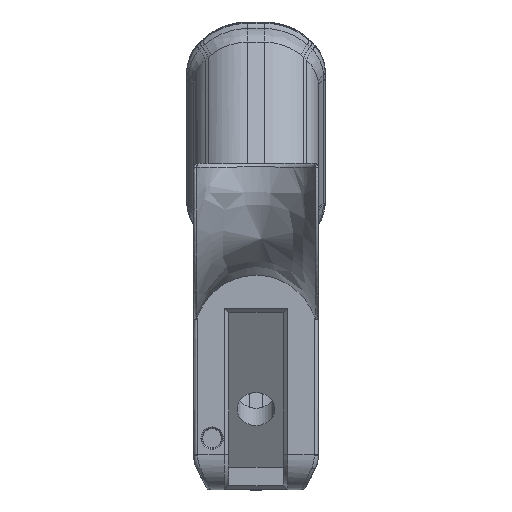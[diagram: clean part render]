
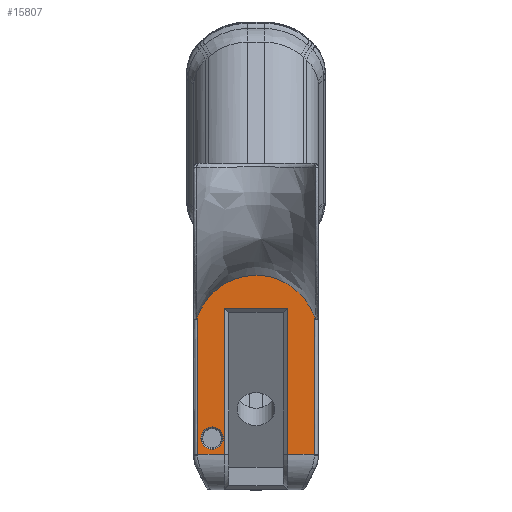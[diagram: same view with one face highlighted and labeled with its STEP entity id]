
A CAD part, top view. The second image highlights one B-rep face of the part: STEP entity #15807.
In plain terms, the highlighted planar face has unit normal (0, 0, 1).
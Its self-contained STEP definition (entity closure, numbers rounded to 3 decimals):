
#673=B_SPLINE_CURVE_WITH_KNOTS('',3,(#37954,#37955,#37956,#37957,#37958,
#37959,#37960,#37961,#37962,#37963,#37964,#37965),.UNSPECIFIED.,.F.,.F.,
(4,2,2,2,2,4),(1.71,1.762,2.19,2.624,
3.022,3.106),.UNSPECIFIED.);
#674=B_SPLINE_CURVE_WITH_KNOTS('',3,(#37967,#37968,#37969,#37970,#37971,
#37972,#37973,#37974,#37975,#37976),.UNSPECIFIED.,.F.,.F.,(4,2,2,2,4),(0.313,
0.444,0.89,1.331,1.71),
 .UNSPECIFIED.);
#727=B_SPLINE_CURVE_WITH_KNOTS('',3,(#39650,#39651,#39652,#39653),
 .UNSPECIFIED.,.F.,.F.,(4,4),(-2.445,-0.005),
 .UNSPECIFIED.);
#729=B_SPLINE_CURVE_WITH_KNOTS('',3,(#39761,#39762,#39763,#39764),
 .UNSPECIFIED.,.F.,.F.,(4,4),(-7.406,-4.966),
 .UNSPECIFIED.);
#1639=FACE_BOUND('',#4707,.T.);
#2454=CIRCLE('',#17283,2.);
#3603=FACE_OUTER_BOUND('',#4706,.T.);
#4706=EDGE_LOOP('',(#14201,#14202,#14203,#14204,#14205,#14206,#14207,#14208,
#14209));
#4707=EDGE_LOOP('',(#14210));
#5472=LINE('',#37829,#6207);
#5478=LINE('',#37840,#6213);
#5483=LINE('',#37858,#6218);
#5490=LINE('',#39758,#6225);
#5491=LINE('',#39760,#6226);
#6207=VECTOR('',#20745,10.);
#6213=VECTOR('',#20755,10.);
#6218=VECTOR('',#20768,10.);
#6225=VECTOR('',#20829,10.);
#6226=VECTOR('',#20830,10.);
#7397=VERTEX_POINT('',#37827);
#7398=VERTEX_POINT('',#37828);
#7401=VERTEX_POINT('',#37839);
#7405=VERTEX_POINT('',#37857);
#7412=VERTEX_POINT('',#37948);
#7413=VERTEX_POINT('',#37953);
#7414=VERTEX_POINT('',#37966);
#7460=VERTEX_POINT('',#39757);
#7461=VERTEX_POINT('',#39759);
#7462=VERTEX_POINT('',#39765);
#9639=EDGE_CURVE('',#7397,#7398,#5472,.T.);
#9645=EDGE_CURVE('',#7401,#7397,#5478,.T.);
#9652=EDGE_CURVE('',#7405,#7398,#5483,.T.);
#9660=EDGE_CURVE('',#7413,#7412,#673,.T.);
#9661=EDGE_CURVE('',#7414,#7413,#674,.T.);
#9738=EDGE_CURVE('',#7405,#7412,#727,.T.);
#9740=EDGE_CURVE('',#7460,#7401,#5490,.T.);
#9741=EDGE_CURVE('',#7461,#7460,#5491,.T.);
#9742=EDGE_CURVE('',#7414,#7461,#729,.T.);
#9743=EDGE_CURVE('',#7462,#7462,#2454,.T.);
#14201=ORIENTED_EDGE('',*,*,#9660,.T.);
#14202=ORIENTED_EDGE('',*,*,#9738,.F.);
#14203=ORIENTED_EDGE('',*,*,#9652,.T.);
#14204=ORIENTED_EDGE('',*,*,#9639,.F.);
#14205=ORIENTED_EDGE('',*,*,#9645,.F.);
#14206=ORIENTED_EDGE('',*,*,#9740,.F.);
#14207=ORIENTED_EDGE('',*,*,#9741,.F.);
#14208=ORIENTED_EDGE('',*,*,#9742,.F.);
#14209=ORIENTED_EDGE('',*,*,#9661,.T.);
#14210=ORIENTED_EDGE('',*,*,#9743,.F.);
#14774=PLANE('',#17282);
#15807=ADVANCED_FACE('',(#3603,#1639),#14774,.T.);
#17282=AXIS2_PLACEMENT_3D('',#39756,#20827,#20828);
#17283=AXIS2_PLACEMENT_3D('',#39766,#20831,#20832);
#20745=DIRECTION('',(0.,-1.,0.));
#20755=DIRECTION('',(-1.,0.,0.));
#20768=DIRECTION('',(1.,0.,0.));
#20827=DIRECTION('center_axis',(0.,0.,
1.));
#20828=DIRECTION('ref_axis',(0.,-1.,0.));
#20829=DIRECTION('',(0.,1.,0.));
#20830=DIRECTION('',(-1.,0.,0.));
#20831=DIRECTION('center_axis',(0.,0.,
1.));
#20832=DIRECTION('ref_axis',(1.,0.,0.));
#37827=CARTESIAN_POINT('',(18.417,-117.318,28.406));
#37828=CARTESIAN_POINT('',(18.417,-143.468,28.406));
#37829=CARTESIAN_POINT('',(18.417,-114.618,28.406));
#37839=CARTESIAN_POINT('',(29.746,-117.318,28.406));
#37840=CARTESIAN_POINT('',(24.173,-117.318,28.406));
#37857=CARTESIAN_POINT('',(13.65,-143.468,28.406));
#37858=CARTESIAN_POINT('',(28.956,-143.468,28.406));
#37948=CARTESIAN_POINT('',(13.518,-119.073,28.406));
#37953=CARTESIAN_POINT('',(24.081,-111.416,28.406));
#37954=CARTESIAN_POINT('Ctrl Pts',(24.081,-111.416,28.406));
#37955=CARTESIAN_POINT('Ctrl Pts',(23.907,-111.416,28.406));
#37956=CARTESIAN_POINT('Ctrl Pts',(23.733,-111.42,28.406));
#37957=CARTESIAN_POINT('Ctrl Pts',(22.136,-111.497,28.406));
#37958=CARTESIAN_POINT('Ctrl Pts',(20.743,-111.842,28.406));
#37959=CARTESIAN_POINT('Ctrl Pts',(18.138,-113.053,28.406));
#37960=CARTESIAN_POINT('Ctrl Pts',(16.956,-113.915,28.406));
#37961=CARTESIAN_POINT('Ctrl Pts',(15.066,-115.943,28.406));
#37962=CARTESIAN_POINT('Ctrl Pts',(14.34,-117.063,28.406));
#37963=CARTESIAN_POINT('Ctrl Pts',(13.71,-118.541,28.406));
#37964=CARTESIAN_POINT('Ctrl Pts',(13.609,-118.805,28.406));
#37965=CARTESIAN_POINT('Ctrl Pts',(13.518,-119.073,28.406));
#37966=CARTESIAN_POINT('',(34.645,-119.073,28.406));
#37967=CARTESIAN_POINT('Ctrl Pts',(34.645,-119.073,28.406));
#37968=CARTESIAN_POINT('Ctrl Pts',(34.504,-118.659,28.406));
#37969=CARTESIAN_POINT('Ctrl Pts',(34.339,-118.252,28.406));
#37970=CARTESIAN_POINT('Ctrl Pts',(33.514,-116.514,28.406));
#37971=CARTESIAN_POINT('Ctrl Pts',(32.621,-115.308,28.406));
#37972=CARTESIAN_POINT('Ctrl Pts',(30.434,-113.323,28.406));
#37973=CARTESIAN_POINT('Ctrl Pts',(29.164,-112.556,28.406));
#37974=CARTESIAN_POINT('Ctrl Pts',(26.592,-111.634,28.406));
#37975=CARTESIAN_POINT('Ctrl Pts',(25.341,-111.416,28.406));
#37976=CARTESIAN_POINT('Ctrl Pts',(24.081,-111.416,28.406));
#39650=CARTESIAN_POINT('Ctrl Pts',(13.65,-143.468,28.406));
#39651=CARTESIAN_POINT('Ctrl Pts',(13.606,-135.336,28.406));
#39652=CARTESIAN_POINT('Ctrl Pts',(13.562,-127.206,28.406));
#39653=CARTESIAN_POINT('Ctrl Pts',(13.518,-119.073,28.406));
#39756=CARTESIAN_POINT('Origin',(19.207,-112.624,28.406));
#39757=CARTESIAN_POINT('',(29.746,-143.468,28.406));
#39758=CARTESIAN_POINT('',(29.746,-114.618,28.406));
#39759=CARTESIAN_POINT('',(34.513,-143.468,28.406));
#39760=CARTESIAN_POINT('',(19.207,-143.468,28.406));
#39761=CARTESIAN_POINT('Ctrl Pts',(34.645,-119.073,28.406));
#39762=CARTESIAN_POINT('Ctrl Pts',(34.601,-127.206,28.406));
#39763=CARTESIAN_POINT('Ctrl Pts',(34.557,-135.336,28.406));
#39764=CARTESIAN_POINT('Ctrl Pts',(34.513,-143.468,28.406));
#39765=CARTESIAN_POINT('',(14.205,-140.572,28.406));
#39766=CARTESIAN_POINT('Origin',(16.205,-140.572,28.406));
